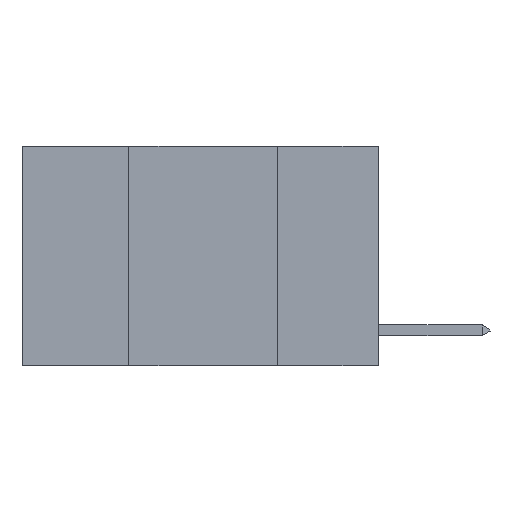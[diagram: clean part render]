
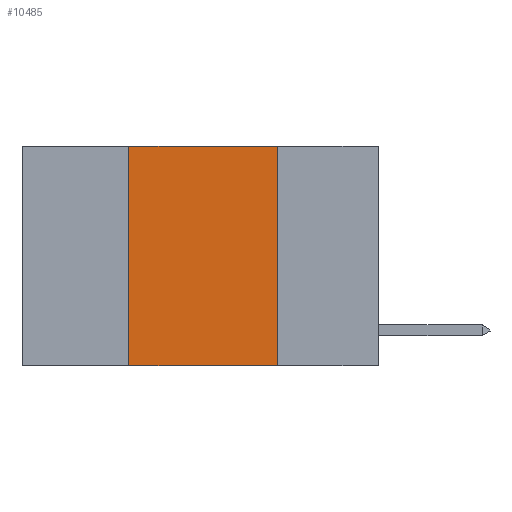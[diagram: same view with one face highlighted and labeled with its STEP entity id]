
A CAD part, left-side view. The second image highlights one B-rep face of the part: STEP entity #10485.
In plain terms, the highlighted planar face has unit normal (-1, 0, 0).
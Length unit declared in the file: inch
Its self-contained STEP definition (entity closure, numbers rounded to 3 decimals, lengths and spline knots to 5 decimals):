
#461 = VECTOR ( 'NONE', #9022, 39.37008 ) ;
#775 = LINE ( 'NONE', #7818, #11344 ) ;
#808 = LINE ( 'NONE', #2846, #461 ) ;
#1066 = VERTEX_POINT ( 'NONE', #6318 ) ;
#1774 = EDGE_CURVE ( 'NONE', #7774, #2688, #775, .T. ) ;
#1786 = EDGE_CURVE ( 'NONE', #1066, #6479, #9129, .T. ) ;
#1817 = AXIS2_PLACEMENT_3D ( 'NONE', #11180, #5285, #12124 ) ;
#2688 = VERTEX_POINT ( 'NONE', #11630 ) ;
#2846 = CARTESIAN_POINT ( 'NONE',  ( 0., 0.17, 0. ) ) ;
#3123 = ORIENTED_EDGE ( 'NONE', *, *, #11510, .F. ) ;
#3445 = ORIENTED_EDGE ( 'NONE', *, *, #1774, .F. ) ;
#3695 = VECTOR ( 'NONE', #12033, 39.37008 ) ;
#4733 = VECTOR ( 'NONE', #9023, 39.37008 ) ;
#4769 = FACE_OUTER_BOUND ( 'NONE', #12937, .T. ) ;
#5285 = DIRECTION ( 'NONE',  ( 1., 0., 0. ) ) ;
#6318 = CARTESIAN_POINT ( 'NONE',  ( 0., 0.42, -0.37 ) ) ;
#6479 = VERTEX_POINT ( 'NONE', #13016 ) ;
#6600 = ORIENTED_EDGE ( 'NONE', *, *, #7398, .F. ) ;
#7398 = EDGE_CURVE ( 'NONE', #1066, #7774, #7447, .T. ) ;
#7447 = LINE ( 'NONE', #8990, #4733 ) ;
#7724 = CARTESIAN_POINT ( 'NONE',  ( 0., 0.42, 0. ) ) ;
#7774 = VERTEX_POINT ( 'NONE', #7724 ) ;
#7818 = CARTESIAN_POINT ( 'NONE',  ( 0., 0.6, 0. ) ) ;
#8990 = CARTESIAN_POINT ( 'NONE',  ( 0., 0.42, 0. ) ) ;
#9022 = DIRECTION ( 'NONE',  ( 0., 0., -1. ) ) ;
#9023 = DIRECTION ( 'NONE',  ( 0., 0., 1. ) ) ;
#9129 = LINE ( 'NONE', #12858, #3695 ) ;
#9219 = ORIENTED_EDGE ( 'NONE', *, *, #1786, .T. ) ;
#10174 = PLANE ( 'NONE',  #1817 ) ;
#10485 = ADVANCED_FACE ( 'NONE', ( #4769 ), #10174, .F. ) ;
#11180 = CARTESIAN_POINT ( 'NONE',  ( 0., 0.6, 0. ) ) ;
#11344 = VECTOR ( 'NONE', #12486, 39.37008 ) ;
#11510 = EDGE_CURVE ( 'NONE', #2688, #6479, #808, .T. ) ;
#11630 = CARTESIAN_POINT ( 'NONE',  ( 0., 0.17, 0. ) ) ;
#12033 = DIRECTION ( 'NONE',  ( 0., -1., 0. ) ) ;
#12124 = DIRECTION ( 'NONE',  ( 0., 0., -1. ) ) ;
#12486 = DIRECTION ( 'NONE',  ( 0., -1., 0. ) ) ;
#12858 = CARTESIAN_POINT ( 'NONE',  ( 0., 0.6, -0.37 ) ) ;
#12937 = EDGE_LOOP ( 'NONE', ( #3123, #3445, #6600, #9219 ) ) ;
#13016 = CARTESIAN_POINT ( 'NONE',  ( 0., 0.17, -0.37 ) ) ;
